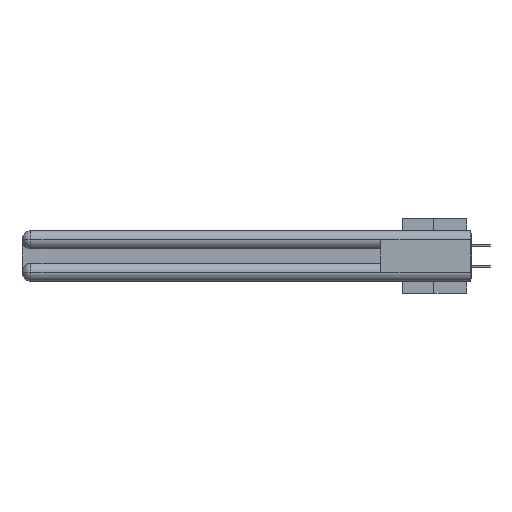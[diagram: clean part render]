
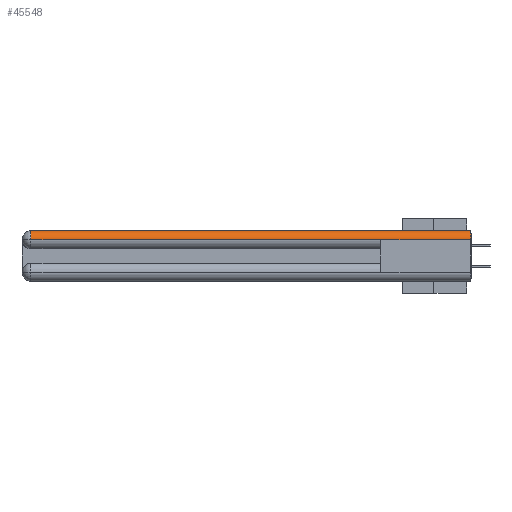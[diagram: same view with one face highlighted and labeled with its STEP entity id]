
A CAD part, left-side view. The second image highlights one B-rep face of the part: STEP entity #45548.
In plain terms, the highlighted cylindrical face has radius 1.562 mm (diameter 3.124 mm), a partial arc.
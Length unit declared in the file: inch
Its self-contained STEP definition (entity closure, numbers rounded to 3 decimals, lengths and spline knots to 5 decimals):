
#146 = CARTESIAN_POINT ( 'NONE',  ( 0.0615, 0., -0.0615 ) ) ;
#1171 = AXIS2_PLACEMENT_3D ( 'NONE', #35441, #31131, #16292 ) ;
#3850 = VERTEX_POINT ( 'NONE', #10354 ) ;
#4235 = VERTEX_POINT ( 'NONE', #18714 ) ;
#4714 = VERTEX_POINT ( 'NONE', #35301 ) ;
#5356 = EDGE_CURVE ( 'NONE', #4235, #4714, #29493, .T. ) ;
#6668 = EDGE_CURVE ( 'NONE', #3850, #4235, #48296, .T. ) ;
#7964 = LINE ( 'NONE', #39564, #40480 ) ;
#8282 = CARTESIAN_POINT ( 'NONE',  ( 0., 3., -0.0615 ) ) ;
#8893 = EDGE_CURVE ( 'NONE', #44083, #37729, #10129, .T. ) ;
#10129 = CIRCLE ( 'NONE', #1171, 0.0615 ) ;
#10354 = CARTESIAN_POINT ( 'NONE',  ( 0.0615, 2.94, 0. ) ) ;
#10582 = AXIS2_PLACEMENT_3D ( 'NONE', #20320, #27253, #35008 ) ;
#14455 = ORIENTED_EDGE ( 'NONE', *, *, #41636, .F. ) ;
#14962 = ORIENTED_EDGE ( 'NONE', *, *, #38196, .F. ) ;
#15569 = FACE_OUTER_BOUND ( 'NONE', #18106, .T. ) ;
#16292 = DIRECTION ( 'NONE',  ( 1., 0., 0. ) ) ;
#18106 = EDGE_LOOP ( 'NONE', ( #14962, #29548, #23095, #14455, #41320 ) ) ;
#18541 = CYLINDRICAL_SURFACE ( 'NONE', #48832, 0.0615 ) ;
#18714 = CARTESIAN_POINT ( 'NONE',  ( 0., 2.94, -0.0615 ) ) ;
#20320 = CARTESIAN_POINT ( 'NONE',  ( 0.0615, 2.94, -0.0615 ) ) ;
#23074 = DIRECTION ( 'NONE',  ( 0., 0., 1. ) ) ;
#23095 = ORIENTED_EDGE ( 'NONE', *, *, #5356, .T. ) ;
#23219 = VECTOR ( 'NONE', #42254, 39.37008 ) ;
#24472 = DIRECTION ( 'NONE',  ( 0., -1., 0. ) ) ;
#27253 = DIRECTION ( 'NONE',  ( 0., -1., 0. ) ) ;
#29493 = LINE ( 'NONE', #42700, #38954 ) ;
#29548 = ORIENTED_EDGE ( 'NONE', *, *, #6668, .T. ) ;
#31131 = DIRECTION ( 'NONE',  ( 0., -1., 0. ) ) ;
#35008 = DIRECTION ( 'NONE',  ( 0., 0., 1. ) ) ;
#35301 = CARTESIAN_POINT ( 'NONE',  ( 0., 0.6, -0.0615 ) ) ;
#35440 = CARTESIAN_POINT ( 'NONE',  ( 0., 0., -0.0615 ) ) ;
#35441 = CARTESIAN_POINT ( 'NONE',  ( 0.0615, 0., -0.0615 ) ) ;
#37729 = VERTEX_POINT ( 'NONE', #35440 ) ;
#38196 = EDGE_CURVE ( 'NONE', #3850, #44083, #7964, .T. ) ;
#38461 = DIRECTION ( 'NONE',  ( 0., -1., 0. ) ) ;
#38954 = VECTOR ( 'NONE', #38461, 39.37008 ) ;
#39247 = LINE ( 'NONE', #8282, #23219 ) ;
#39564 = CARTESIAN_POINT ( 'NONE',  ( 0.0615, 0., 0. ) ) ;
#40480 = VECTOR ( 'NONE', #24472, 39.37008 ) ;
#40813 = CARTESIAN_POINT ( 'NONE',  ( 0.0615, 0., 0. ) ) ;
#41320 = ORIENTED_EDGE ( 'NONE', *, *, #8893, .F. ) ;
#41636 = EDGE_CURVE ( 'NONE', #37729, #4714, #39247, .T. ) ;
#42254 = DIRECTION ( 'NONE',  ( 0., 1., 0. ) ) ;
#42700 = CARTESIAN_POINT ( 'NONE',  ( 0., 3., -0.0615 ) ) ;
#44083 = VERTEX_POINT ( 'NONE', #40813 ) ;
#45246 = DIRECTION ( 'NONE',  ( 0., 1., 0. ) ) ;
#45548 = ADVANCED_FACE ( 'NONE', ( #15569 ), #18541, .T. ) ;
#48296 = CIRCLE ( 'NONE', #10582, 0.0615 ) ;
#48832 = AXIS2_PLACEMENT_3D ( 'NONE', #146, #45246, #23074 ) ;
